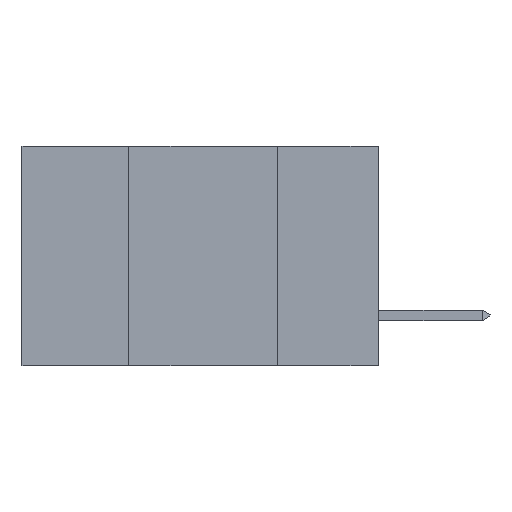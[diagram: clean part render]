
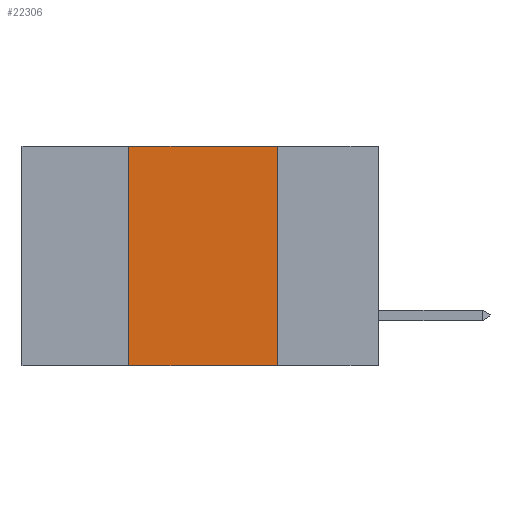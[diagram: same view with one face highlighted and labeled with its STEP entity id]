
A CAD part, left-side view. The second image highlights one B-rep face of the part: STEP entity #22306.
In plain terms, the highlighted planar face has unit normal (-1, 0, 0).
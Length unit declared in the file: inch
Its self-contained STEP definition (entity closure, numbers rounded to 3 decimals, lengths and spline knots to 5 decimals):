
#463 = ORIENTED_EDGE ( 'NONE', *, *, #23830, .F. ) ;
#465 = DIRECTION ( 'NONE',  ( 0., 0., 1. ) ) ;
#778 = LINE ( 'NONE', #30035, #18735 ) ;
#1015 = PLANE ( 'NONE',  #28040 ) ;
#1229 = FACE_OUTER_BOUND ( 'NONE', #20799, .T. ) ;
#1554 = VECTOR ( 'NONE', #13476, 39.37008 ) ;
#5559 = CARTESIAN_POINT ( 'NONE',  ( 0., 0.17, 0. ) ) ;
#7682 = EDGE_CURVE ( 'NONE', #30083, #9421, #15813, .T. ) ;
#7941 = DIRECTION ( 'NONE',  ( 0., 0., -1. ) ) ;
#9355 = VERTEX_POINT ( 'NONE', #19166 ) ;
#9421 = VERTEX_POINT ( 'NONE', #28670 ) ;
#9638 = VECTOR ( 'NONE', #7941, 39.37008 ) ;
#9872 = CARTESIAN_POINT ( 'NONE',  ( 0., 0.42, 0. ) ) ;
#12859 = DIRECTION ( 'NONE',  ( 1., 0., 0. ) ) ;
#12958 = ORIENTED_EDGE ( 'NONE', *, *, #28520, .T. ) ;
#13476 = DIRECTION ( 'NONE',  ( 0., -1., 0. ) ) ;
#14549 = ORIENTED_EDGE ( 'NONE', *, *, #7682, .F. ) ;
#15263 = VERTEX_POINT ( 'NONE', #23757 ) ;
#15813 = LINE ( 'NONE', #5559, #9638 ) ;
#16280 = DIRECTION ( 'NONE',  ( 0., -1., 0. ) ) ;
#18735 = VECTOR ( 'NONE', #16280, 39.37008 ) ;
#19166 = CARTESIAN_POINT ( 'NONE',  ( 0., 0.42, 0. ) ) ;
#20799 = EDGE_LOOP ( 'NONE', ( #14549, #29221, #463, #12958 ) ) ;
#21686 = LINE ( 'NONE', #29655, #1554 ) ;
#22146 = CARTESIAN_POINT ( 'NONE',  ( 0., 0.17, 0. ) ) ;
#22306 = ADVANCED_FACE ( 'NONE', ( #1229 ), #1015, .F. ) ;
#22365 = VECTOR ( 'NONE', #465, 39.37008 ) ;
#23503 = EDGE_CURVE ( 'NONE', #9355, #30083, #21686, .T. ) ;
#23757 = CARTESIAN_POINT ( 'NONE',  ( 0., 0.42, -0.37 ) ) ;
#23830 = EDGE_CURVE ( 'NONE', #15263, #9355, #28532, .T. ) ;
#26699 = CARTESIAN_POINT ( 'NONE',  ( 0., 0.6, 0. ) ) ;
#28040 = AXIS2_PLACEMENT_3D ( 'NONE', #26699, #12859, #29032 ) ;
#28520 = EDGE_CURVE ( 'NONE', #15263, #9421, #778, .T. ) ;
#28532 = LINE ( 'NONE', #9872, #22365 ) ;
#28670 = CARTESIAN_POINT ( 'NONE',  ( 0., 0.17, -0.37 ) ) ;
#29032 = DIRECTION ( 'NONE',  ( 0., 0., -1. ) ) ;
#29221 = ORIENTED_EDGE ( 'NONE', *, *, #23503, .F. ) ;
#29655 = CARTESIAN_POINT ( 'NONE',  ( 0., 0.6, 0. ) ) ;
#30035 = CARTESIAN_POINT ( 'NONE',  ( 0., 0.6, -0.37 ) ) ;
#30083 = VERTEX_POINT ( 'NONE', #22146 ) ;
